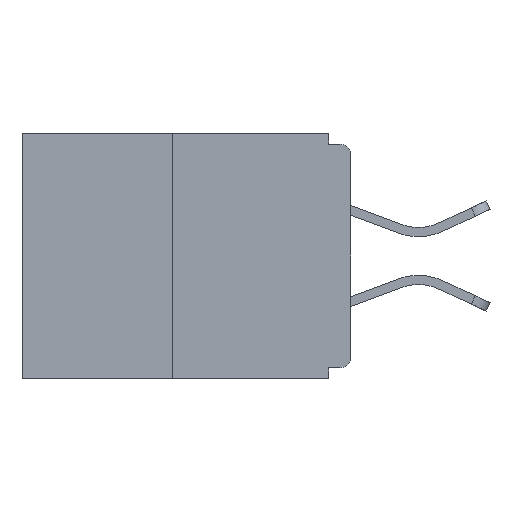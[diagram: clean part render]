
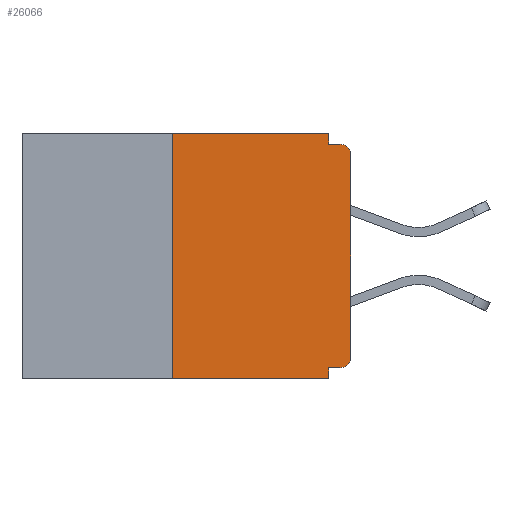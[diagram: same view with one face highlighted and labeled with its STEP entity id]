
A CAD part, left-side view. The second image highlights one B-rep face of the part: STEP entity #26066.
In plain terms, the highlighted planar face has unit normal (-1, 0, 0).
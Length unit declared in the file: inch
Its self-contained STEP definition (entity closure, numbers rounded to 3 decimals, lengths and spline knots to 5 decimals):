
#430 = VERTEX_POINT ( 'NONE', #4275 ) ;
#1025 = DIRECTION ( 'NONE',  ( 0., -1., 0. ) ) ;
#1133 = CARTESIAN_POINT ( 'NONE',  ( 0., 0., -0.015 ) ) ;
#1322 = VERTEX_POINT ( 'NONE', #20107 ) ;
#1585 = CARTESIAN_POINT ( 'NONE',  ( 0., 0.015, -0.03 ) ) ;
#1888 = ORIENTED_EDGE ( 'NONE', *, *, #25409, .T. ) ;
#2087 = EDGE_CURVE ( 'NONE', #15511, #430, #6672, .T. ) ;
#2430 = ORIENTED_EDGE ( 'NONE', *, *, #4486, .T. ) ;
#2604 = AXIS2_PLACEMENT_3D ( 'NONE', #1585, #3892, #8277 ) ;
#3392 = CARTESIAN_POINT ( 'NONE',  ( 0., 0.015, -0.015 ) ) ;
#3445 = LINE ( 'NONE', #25919, #24987 ) ;
#3456 = DIRECTION ( 'NONE',  ( 0., 0., -1. ) ) ;
#3837 = EDGE_CURVE ( 'NONE', #10515, #4340, #23255, .T. ) ;
#3892 = DIRECTION ( 'NONE',  ( -1., 0., 0. ) ) ;
#4275 = CARTESIAN_POINT ( 'NONE',  ( 0., 0.25, 0. ) ) ;
#4340 = VERTEX_POINT ( 'NONE', #3392 ) ;
#4486 = EDGE_CURVE ( 'NONE', #1322, #4340, #5240, .T. ) ;
#5240 = CIRCLE ( 'NONE', #2604, 0.015 ) ;
#5476 = CARTESIAN_POINT ( 'NONE',  ( 0., 0.031, -0.015 ) ) ;
#6672 = LINE ( 'NONE', #18894, #12780 ) ;
#6950 = ORIENTED_EDGE ( 'NONE', *, *, #20943, .F. ) ;
#7005 = ORIENTED_EDGE ( 'NONE', *, *, #7269, .T. ) ;
#7269 = EDGE_CURVE ( 'NONE', #19062, #29008, #23340, .T. ) ;
#7337 = VERTEX_POINT ( 'NONE', #13060 ) ;
#7465 = CARTESIAN_POINT ( 'NONE',  ( 0., 0.46, 0. ) ) ;
#8277 = DIRECTION ( 'NONE',  ( 0., 0., -1. ) ) ;
#8353 = ORIENTED_EDGE ( 'NONE', *, *, #2087, .F. ) ;
#8469 = CARTESIAN_POINT ( 'NONE',  ( 0., 0.25, -0.343 ) ) ;
#8913 = VECTOR ( 'NONE', #1025, 39.37008 ) ;
#9243 = DIRECTION ( 'NONE',  ( 0., 1., 0. ) ) ;
#9462 = DIRECTION ( 'NONE',  ( 0., -1., 0. ) ) ;
#9976 = VECTOR ( 'NONE', #9243, 39.37008 ) ;
#10157 = DIRECTION ( 'NONE',  ( 0., -1., 0. ) ) ;
#10515 = VERTEX_POINT ( 'NONE', #5476 ) ;
#10695 = LINE ( 'NONE', #18373, #9976 ) ;
#12275 = DIRECTION ( 'NONE',  ( 0., 0., 1. ) ) ;
#12780 = VECTOR ( 'NONE', #16685, 39.37008 ) ;
#13060 = CARTESIAN_POINT ( 'NONE',  ( 0., 0.031, 0. ) ) ;
#13179 = EDGE_CURVE ( 'NONE', #17974, #14985, #29762, .T. ) ;
#14285 = PLANE ( 'NONE',  #28401 ) ;
#14985 = VERTEX_POINT ( 'NONE', #19824 ) ;
#15511 = VERTEX_POINT ( 'NONE', #8469 ) ;
#15559 = ORIENTED_EDGE ( 'NONE', *, *, #13179, .F. ) ;
#16135 = CARTESIAN_POINT ( 'NONE',  ( 0., 0.031, -0.328 ) ) ;
#16685 = DIRECTION ( 'NONE',  ( 0., 0., 1. ) ) ;
#16904 = ORIENTED_EDGE ( 'NONE', *, *, #28590, .F. ) ;
#17008 = DIRECTION ( 'NONE',  ( 0., 0., -1. ) ) ;
#17115 = CARTESIAN_POINT ( 'NONE',  ( 0., 0., 0. ) ) ;
#17183 = DIRECTION ( 'NONE',  ( -1., 0., 0. ) ) ;
#17974 = VERTEX_POINT ( 'NONE', #16135 ) ;
#18082 = VECTOR ( 'NONE', #9462, 39.37008 ) ;
#18373 = CARTESIAN_POINT ( 'NONE',  ( 0., 0., -0.328 ) ) ;
#18704 = DIRECTION ( 'NONE',  ( 0., 0., -1. ) ) ;
#18894 = CARTESIAN_POINT ( 'NONE',  ( 0., 0.25, 0. ) ) ;
#19062 = VERTEX_POINT ( 'NONE', #29691 ) ;
#19530 = AXIS2_PLACEMENT_3D ( 'NONE', #28541, #17183, #3456 ) ;
#19623 = ORIENTED_EDGE ( 'NONE', *, *, #3837, .F. ) ;
#19824 = CARTESIAN_POINT ( 'NONE',  ( 0., 0.031, -0.343 ) ) ;
#20107 = CARTESIAN_POINT ( 'NONE',  ( 0., 0., -0.03 ) ) ;
#20686 = EDGE_CURVE ( 'NONE', #19062, #17974, #10695, .T. ) ;
#20943 = EDGE_CURVE ( 'NONE', #7337, #10515, #21056, .T. ) ;
#21056 = LINE ( 'NONE', #29229, #24703 ) ;
#22320 = VECTOR ( 'NONE', #12275, 39.37008 ) ;
#23063 = LINE ( 'NONE', #23090, #18082 ) ;
#23090 = CARTESIAN_POINT ( 'NONE',  ( 0., 0.46, -0.343 ) ) ;
#23255 = LINE ( 'NONE', #1133, #8913 ) ;
#23340 = CIRCLE ( 'NONE', #19530, 0.015 ) ;
#23771 = CARTESIAN_POINT ( 'NONE',  ( 0., 0., -0.313 ) ) ;
#24491 = DIRECTION ( 'NONE',  ( 0., 0., -1. ) ) ;
#24703 = VECTOR ( 'NONE', #24491, 39.37008 ) ;
#24896 = ORIENTED_EDGE ( 'NONE', *, *, #20686, .F. ) ;
#24987 = VECTOR ( 'NONE', #10157, 39.37008 ) ;
#25228 = LINE ( 'NONE', #17115, #22320 ) ;
#25409 = EDGE_CURVE ( 'NONE', #15511, #14985, #23063, .T. ) ;
#25429 = VECTOR ( 'NONE', #17008, 39.37008 ) ;
#25852 = DIRECTION ( 'NONE',  ( 1., 0., 0. ) ) ;
#25919 = CARTESIAN_POINT ( 'NONE',  ( 0., 0.46, 0. ) ) ;
#26055 = CARTESIAN_POINT ( 'NONE',  ( 0., 0.031, -0.343 ) ) ;
#26066 = ADVANCED_FACE ( 'NONE', ( #26288 ), #14285, .F. ) ;
#26225 = EDGE_CURVE ( 'NONE', #29008, #1322, #25228, .T. ) ;
#26259 = EDGE_LOOP ( 'NONE', ( #16904, #8353, #1888, #15559, #24896, #7005, #29437, #2430, #19623, #6950 ) ) ;
#26288 = FACE_OUTER_BOUND ( 'NONE', #26259, .T. ) ;
#28401 = AXIS2_PLACEMENT_3D ( 'NONE', #7465, #25852, #18704 ) ;
#28541 = CARTESIAN_POINT ( 'NONE',  ( 0., 0.015, -0.313 ) ) ;
#28590 = EDGE_CURVE ( 'NONE', #430, #7337, #3445, .T. ) ;
#29008 = VERTEX_POINT ( 'NONE', #23771 ) ;
#29229 = CARTESIAN_POINT ( 'NONE',  ( 0., 0.031, 0. ) ) ;
#29437 = ORIENTED_EDGE ( 'NONE', *, *, #26225, .T. ) ;
#29691 = CARTESIAN_POINT ( 'NONE',  ( 0., 0.015, -0.328 ) ) ;
#29762 = LINE ( 'NONE', #26055, #25429 ) ;
